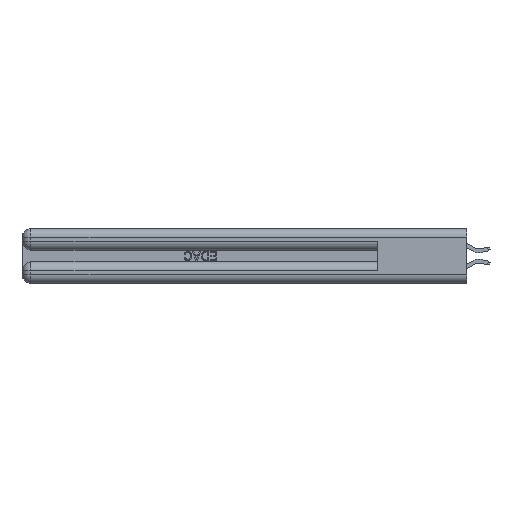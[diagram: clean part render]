
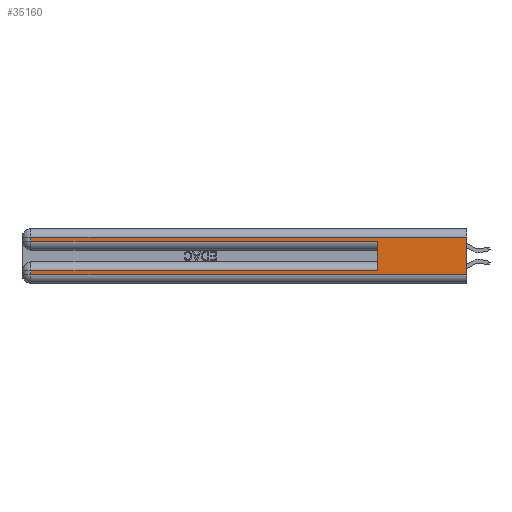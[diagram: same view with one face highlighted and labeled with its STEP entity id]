
A CAD part, left-side view. The second image highlights one B-rep face of the part: STEP entity #35160.
In plain terms, the highlighted planar face has unit normal (-1, 0, 0).
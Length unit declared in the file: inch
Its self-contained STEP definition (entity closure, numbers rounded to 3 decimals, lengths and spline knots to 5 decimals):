
#107 = VERTEX_POINT ( 'NONE', #31781 ) ;
#326 = VERTEX_POINT ( 'NONE', #17784 ) ;
#448 = ORIENTED_EDGE ( 'NONE', *, *, #32406, .T. ) ;
#1056 = DIRECTION ( 'NONE',  ( 0., -1., 0. ) ) ;
#1886 = CARTESIAN_POINT ( 'NONE',  ( 0., 0., 0.31 ) ) ;
#2401 = VERTEX_POINT ( 'NONE', #24107 ) ;
#2507 = ORIENTED_EDGE ( 'NONE', *, *, #17561, .T. ) ;
#2536 = DIRECTION ( 'NONE',  ( 0., 1., 0. ) ) ;
#2974 = CARTESIAN_POINT ( 'NONE',  ( 0., 0., 0.285 ) ) ;
#2976 = CARTESIAN_POINT ( 'NONE',  ( 0., 0., 0.06 ) ) ;
#3605 = EDGE_CURVE ( 'NONE', #7250, #41440, #13263, .T. ) ;
#4258 = ORIENTED_EDGE ( 'NONE', *, *, #23812, .T. ) ;
#5973 = ORIENTED_EDGE ( 'NONE', *, *, #27284, .F. ) ;
#5977 = VECTOR ( 'NONE', #6464, 39.37008 ) ;
#6314 = EDGE_CURVE ( 'NONE', #6914, #41440, #42870, .T. ) ;
#6464 = DIRECTION ( 'NONE',  ( 0., -1., 0. ) ) ;
#6472 = CARTESIAN_POINT ( 'NONE',  ( 0., 0., 0.085 ) ) ;
#6914 = VERTEX_POINT ( 'NONE', #35145 ) ;
#7250 = VERTEX_POINT ( 'NONE', #40565 ) ;
#8410 = CARTESIAN_POINT ( 'NONE',  ( 0., 2.94, 0.085 ) ) ;
#9296 = ORIENTED_EDGE ( 'NONE', *, *, #6314, .T. ) ;
#9388 = FACE_OUTER_BOUND ( 'NONE', #14541, .T. ) ;
#10311 = EDGE_CURVE ( 'NONE', #10838, #107, #24608, .T. ) ;
#10781 = VERTEX_POINT ( 'NONE', #8410 ) ;
#10838 = VERTEX_POINT ( 'NONE', #19280 ) ;
#10979 = DIRECTION ( 'NONE',  ( 1., 0., 0. ) ) ;
#10993 = LINE ( 'NONE', #39622, #13176 ) ;
#13176 = VECTOR ( 'NONE', #31064, 39.37008 ) ;
#13263 = LINE ( 'NONE', #21364, #20888 ) ;
#14541 = EDGE_LOOP ( 'NONE', ( #39492, #39200, #14669, #4258, #5973, #448, #2507, #9296 ) ) ;
#14669 = ORIENTED_EDGE ( 'NONE', *, *, #10311, .T. ) ;
#16657 = CARTESIAN_POINT ( 'NONE',  ( 0., 0., 0.06 ) ) ;
#17471 = DIRECTION ( 'NONE',  ( 0., 0., -1. ) ) ;
#17561 = EDGE_CURVE ( 'NONE', #10781, #6914, #10993, .T. ) ;
#17753 = PLANE ( 'NONE',  #36324 ) ;
#17784 = CARTESIAN_POINT ( 'NONE',  ( 0., 0.6, 0.285 ) ) ;
#18799 = DIRECTION ( 'NONE',  ( 0., 1., 0. ) ) ;
#18899 = LINE ( 'NONE', #2974, #5977 ) ;
#19280 = CARTESIAN_POINT ( 'NONE',  ( 0., 2.94, 0.31 ) ) ;
#20888 = VECTOR ( 'NONE', #32041, 39.37008 ) ;
#21364 = CARTESIAN_POINT ( 'NONE',  ( 0., 0., 0.37 ) ) ;
#21453 = VECTOR ( 'NONE', #18799, 39.37008 ) ;
#22082 = LINE ( 'NONE', #6472, #24774 ) ;
#22381 = LINE ( 'NONE', #43814, #30036 ) ;
#23812 = EDGE_CURVE ( 'NONE', #107, #326, #18899, .T. ) ;
#24107 = CARTESIAN_POINT ( 'NONE',  ( 0., 0.6, 0.085 ) ) ;
#24608 = LINE ( 'NONE', #34140, #30632 ) ;
#24626 = CARTESIAN_POINT ( 'NONE',  ( 0., 0., 0.37 ) ) ;
#24774 = VECTOR ( 'NONE', #2536, 39.37008 ) ;
#27153 = VECTOR ( 'NONE', #1056, 39.37008 ) ;
#27284 = EDGE_CURVE ( 'NONE', #2401, #326, #22381, .T. ) ;
#27475 = LINE ( 'NONE', #1886, #21453 ) ;
#29886 = DIRECTION ( 'NONE',  ( 0., 0., 1. ) ) ;
#30036 = VECTOR ( 'NONE', #29886, 39.37008 ) ;
#30632 = VECTOR ( 'NONE', #40648, 39.37008 ) ;
#31064 = DIRECTION ( 'NONE',  ( 0., 0., -1. ) ) ;
#31781 = CARTESIAN_POINT ( 'NONE',  ( 0., 2.94, 0.285 ) ) ;
#32041 = DIRECTION ( 'NONE',  ( 0., 0., -1. ) ) ;
#32406 = EDGE_CURVE ( 'NONE', #2401, #10781, #22082, .T. ) ;
#32938 = EDGE_CURVE ( 'NONE', #7250, #10838, #27475, .T. ) ;
#34140 = CARTESIAN_POINT ( 'NONE',  ( 0., 2.94, 0.37 ) ) ;
#35145 = CARTESIAN_POINT ( 'NONE',  ( 0., 2.94, 0.06 ) ) ;
#35160 = ADVANCED_FACE ( 'NONE', ( #9388 ), #17753, .F. ) ;
#36324 = AXIS2_PLACEMENT_3D ( 'NONE', #24626, #10979, #17471 ) ;
#39200 = ORIENTED_EDGE ( 'NONE', *, *, #32938, .T. ) ;
#39492 = ORIENTED_EDGE ( 'NONE', *, *, #3605, .F. ) ;
#39622 = CARTESIAN_POINT ( 'NONE',  ( 0., 2.94, 0.37 ) ) ;
#40565 = CARTESIAN_POINT ( 'NONE',  ( 0., 0., 0.31 ) ) ;
#40648 = DIRECTION ( 'NONE',  ( 0., 0., -1. ) ) ;
#41440 = VERTEX_POINT ( 'NONE', #2976 ) ;
#42870 = LINE ( 'NONE', #16657, #27153 ) ;
#43814 = CARTESIAN_POINT ( 'NONE',  ( 0., 0.6, 0.145 ) ) ;
